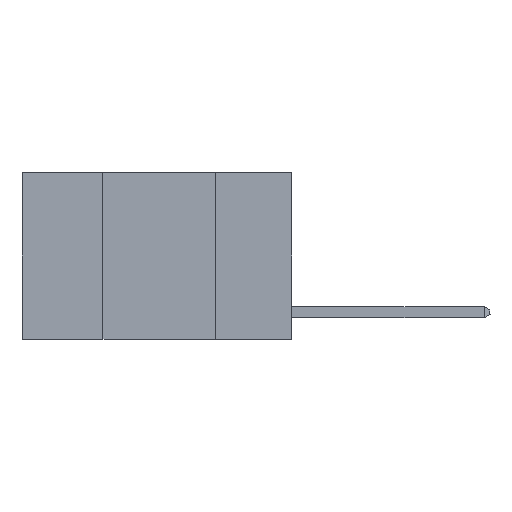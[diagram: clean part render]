
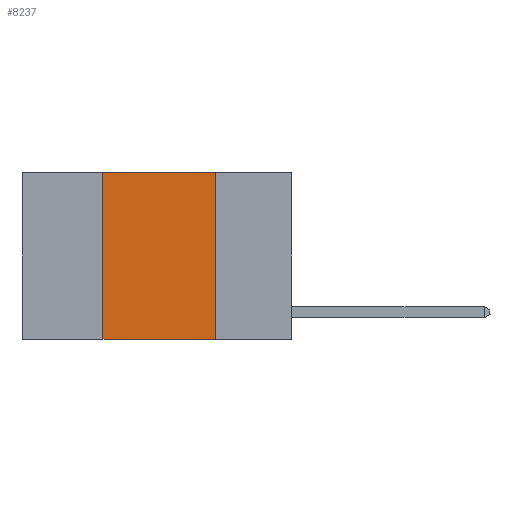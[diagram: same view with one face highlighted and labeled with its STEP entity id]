
A CAD part, left-side view. The second image highlights one B-rep face of the part: STEP entity #8237.
In plain terms, the highlighted planar face has unit normal (-1, 0, 0).
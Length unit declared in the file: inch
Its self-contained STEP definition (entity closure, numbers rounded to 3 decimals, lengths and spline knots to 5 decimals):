
#36 = CARTESIAN_POINT ( 'NONE',  ( 0., 0.17, 0. ) ) ;
#800 = ORIENTED_EDGE ( 'NONE', *, *, #8242, .F. ) ;
#1608 = FACE_OUTER_BOUND ( 'NONE', #6468, .T. ) ;
#1651 = ORIENTED_EDGE ( 'NONE', *, *, #3386, .F. ) ;
#3386 = EDGE_CURVE ( 'NONE', #7363, #16585, #19110, .T. ) ;
#4419 = LINE ( 'NONE', #5199, #8702 ) ;
#4768 = CARTESIAN_POINT ( 'NONE',  ( 0., 0.17, 0. ) ) ;
#5199 = CARTESIAN_POINT ( 'NONE',  ( 0., 0.6, -0.37 ) ) ;
#6382 = CARTESIAN_POINT ( 'NONE',  ( 0., 0.6, 0. ) ) ;
#6468 = EDGE_LOOP ( 'NONE', ( #800, #8339, #1651, #12773 ) ) ;
#7187 = VECTOR ( 'NONE', #8076, 39.37008 ) ;
#7363 = VERTEX_POINT ( 'NONE', #13599 ) ;
#8076 = DIRECTION ( 'NONE',  ( 0., 0., 1. ) ) ;
#8147 = PLANE ( 'NONE',  #8176 ) ;
#8176 = AXIS2_PLACEMENT_3D ( 'NONE', #17875, #18546, #9675 ) ;
#8237 = ADVANCED_FACE ( 'NONE', ( #1608 ), #8147, .F. ) ;
#8242 = EDGE_CURVE ( 'NONE', #10983, #17928, #13664, .T. ) ;
#8339 = ORIENTED_EDGE ( 'NONE', *, *, #8859, .F. ) ;
#8702 = VECTOR ( 'NONE', #12916, 39.37008 ) ;
#8859 = EDGE_CURVE ( 'NONE', #16585, #10983, #19116, .T. ) ;
#9547 = CARTESIAN_POINT ( 'NONE',  ( 0., 0.17, -0.37 ) ) ;
#9610 = DIRECTION ( 'NONE',  ( 0., 0., -1. ) ) ;
#9657 = VECTOR ( 'NONE', #9610, 39.37008 ) ;
#9675 = DIRECTION ( 'NONE',  ( 0., 0., -1. ) ) ;
#10671 = CARTESIAN_POINT ( 'NONE',  ( 0., 0.42, 0. ) ) ;
#10983 = VERTEX_POINT ( 'NONE', #4768 ) ;
#12575 = DIRECTION ( 'NONE',  ( 0., -1., 0. ) ) ;
#12773 = ORIENTED_EDGE ( 'NONE', *, *, #18056, .T. ) ;
#12916 = DIRECTION ( 'NONE',  ( 0., -1., 0. ) ) ;
#13599 = CARTESIAN_POINT ( 'NONE',  ( 0., 0.42, -0.37 ) ) ;
#13664 = LINE ( 'NONE', #36, #9657 ) ;
#14760 = VECTOR ( 'NONE', #12575, 39.37008 ) ;
#15532 = CARTESIAN_POINT ( 'NONE',  ( 0., 0.42, 0. ) ) ;
#16585 = VERTEX_POINT ( 'NONE', #10671 ) ;
#17875 = CARTESIAN_POINT ( 'NONE',  ( 0., 0.6, 0. ) ) ;
#17928 = VERTEX_POINT ( 'NONE', #9547 ) ;
#18056 = EDGE_CURVE ( 'NONE', #7363, #17928, #4419, .T. ) ;
#18546 = DIRECTION ( 'NONE',  ( 1., 0., 0. ) ) ;
#19110 = LINE ( 'NONE', #15532, #7187 ) ;
#19116 = LINE ( 'NONE', #6382, #14760 ) ;
